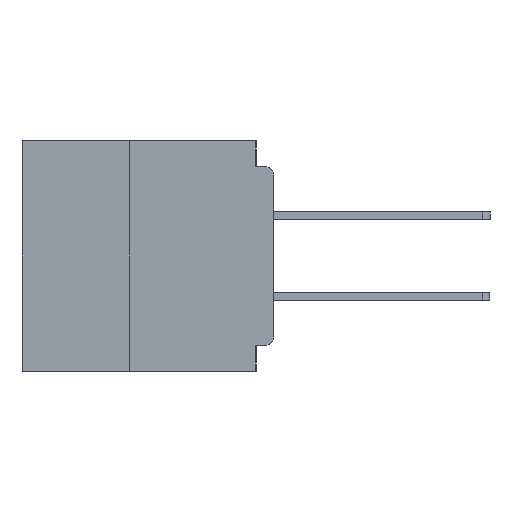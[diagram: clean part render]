
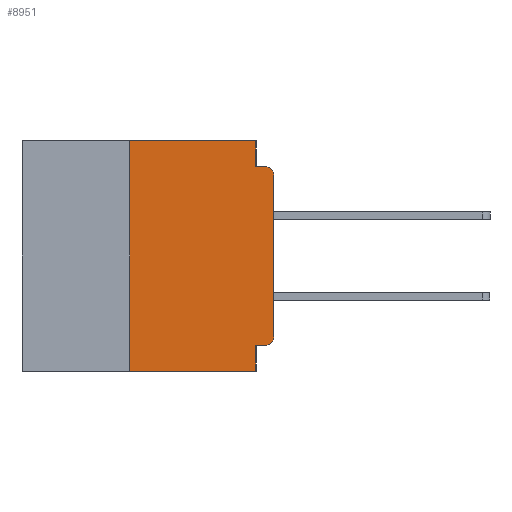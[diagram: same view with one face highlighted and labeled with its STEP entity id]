
A CAD part, left-side view. The second image highlights one B-rep face of the part: STEP entity #8951.
In plain terms, the highlighted planar face has unit normal (-1, 0, 0).
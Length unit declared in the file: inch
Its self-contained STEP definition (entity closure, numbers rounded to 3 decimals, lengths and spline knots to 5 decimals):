
#564 = DIRECTION ( 'NONE',  ( 0., -1., 0. ) ) ;
#827 = VERTEX_POINT ( 'NONE', #9445 ) ;
#1627 = VERTEX_POINT ( 'NONE', #43215 ) ;
#2192 = EDGE_CURVE ( 'NONE', #17711, #7327, #29854, .T. ) ;
#2783 = EDGE_CURVE ( 'NONE', #35785, #17711, #11024, .T. ) ;
#3082 = VECTOR ( 'NONE', #45607, 39.37008 ) ;
#7291 = ORIENTED_EDGE ( 'NONE', *, *, #34549, .F. ) ;
#7327 = VERTEX_POINT ( 'NONE', #21903 ) ;
#8363 = CARTESIAN_POINT ( 'NONE',  ( 0., 0.031, -0.355 ) ) ;
#8951 = ADVANCED_FACE ( 'NONE', ( #32500 ), #48819, .F. ) ;
#9445 = CARTESIAN_POINT ( 'NONE',  ( 0., 0.031, -0.045 ) ) ;
#10559 = VECTOR ( 'NONE', #37713, 39.37008 ) ;
#11024 = LINE ( 'NONE', #31619, #42430 ) ;
#11606 = EDGE_CURVE ( 'NONE', #52556, #18619, #43250, .T. ) ;
#11915 = CARTESIAN_POINT ( 'NONE',  ( 0., 0.437, 0. ) ) ;
#12272 = DIRECTION ( 'NONE',  ( 1., 0., 0. ) ) ;
#12718 = EDGE_CURVE ( 'NONE', #1627, #50601, #43747, .T. ) ;
#13626 = LINE ( 'NONE', #33648, #53060 ) ;
#14675 = VERTEX_POINT ( 'NONE', #44619 ) ;
#15361 = DIRECTION ( 'NONE',  ( 0., 0., 1. ) ) ;
#15692 = ORIENTED_EDGE ( 'NONE', *, *, #11606, .F. ) ;
#15844 = CARTESIAN_POINT ( 'NONE',  ( 0., 0.25, 0. ) ) ;
#17711 = VERTEX_POINT ( 'NONE', #30572 ) ;
#18619 = VERTEX_POINT ( 'NONE', #30398 ) ;
#20416 = CARTESIAN_POINT ( 'NONE',  ( 0., 0., -0.045 ) ) ;
#20626 = ORIENTED_EDGE ( 'NONE', *, *, #25111, .F. ) ;
#21029 = LINE ( 'NONE', #20416, #30584 ) ;
#21414 = LINE ( 'NONE', #23092, #42988 ) ;
#21698 = DIRECTION ( 'NONE',  ( -1., 0., 0. ) ) ;
#21903 = CARTESIAN_POINT ( 'NONE',  ( 0., 0.015, -0.045 ) ) ;
#22174 = VECTOR ( 'NONE', #15361, 39.37008 ) ;
#23092 = CARTESIAN_POINT ( 'NONE',  ( 0., 0., -0.355 ) ) ;
#24499 = EDGE_CURVE ( 'NONE', #50601, #25359, #13626, .T. ) ;
#25111 = EDGE_CURVE ( 'NONE', #25359, #827, #25230, .T. ) ;
#25230 = LINE ( 'NONE', #49822, #3082 ) ;
#25359 = VERTEX_POINT ( 'NONE', #51547 ) ;
#25375 = ORIENTED_EDGE ( 'NONE', *, *, #2783, .T. ) ;
#25551 = AXIS2_PLACEMENT_3D ( 'NONE', #11915, #12272, #40908 ) ;
#26894 = EDGE_CURVE ( 'NONE', #14675, #35785, #45286, .T. ) ;
#28307 = EDGE_CURVE ( 'NONE', #827, #7327, #21029, .T. ) ;
#29206 = VECTOR ( 'NONE', #30000, 39.37008 ) ;
#29854 = CIRCLE ( 'NONE', #42615, 0.015 ) ;
#29859 = EDGE_LOOP ( 'NONE', ( #25375, #40668, #43704, #20626, #52416, #32809, #48382, #15692, #7291, #38996 ) ) ;
#30000 = DIRECTION ( 'NONE',  ( 0., -1., 0. ) ) ;
#30398 = CARTESIAN_POINT ( 'NONE',  ( 0., 0.031, -0.4 ) ) ;
#30572 = CARTESIAN_POINT ( 'NONE',  ( 0., 0., -0.06 ) ) ;
#30584 = VECTOR ( 'NONE', #52757, 39.37008 ) ;
#31582 = DIRECTION ( 'NONE',  ( 0., 0., 1. ) ) ;
#31619 = CARTESIAN_POINT ( 'NONE',  ( 0., 0., 0. ) ) ;
#32500 = FACE_OUTER_BOUND ( 'NONE', #29859, .T. ) ;
#32809 = ORIENTED_EDGE ( 'NONE', *, *, #12718, .F. ) ;
#33648 = CARTESIAN_POINT ( 'NONE',  ( 0., 0.437, 0. ) ) ;
#33652 = CARTESIAN_POINT ( 'NONE',  ( 0., 0.031, -0.4 ) ) ;
#34549 = EDGE_CURVE ( 'NONE', #14675, #52556, #21414, .T. ) ;
#35204 = AXIS2_PLACEMENT_3D ( 'NONE', #45961, #21698, #50005 ) ;
#35780 = CARTESIAN_POINT ( 'NONE',  ( 0., 0.25, -0.4 ) ) ;
#35785 = VERTEX_POINT ( 'NONE', #44868 ) ;
#37713 = DIRECTION ( 'NONE',  ( 0., 0., -1. ) ) ;
#38996 = ORIENTED_EDGE ( 'NONE', *, *, #26894, .T. ) ;
#39945 = LINE ( 'NONE', #42020, #29206 ) ;
#40668 = ORIENTED_EDGE ( 'NONE', *, *, #2192, .T. ) ;
#40908 = DIRECTION ( 'NONE',  ( 0., 0., -1. ) ) ;
#42020 = CARTESIAN_POINT ( 'NONE',  ( 0., 0.437, -0.4 ) ) ;
#42430 = VECTOR ( 'NONE', #31582, 39.37008 ) ;
#42615 = AXIS2_PLACEMENT_3D ( 'NONE', #51393, #51164, #50764 ) ;
#42988 = VECTOR ( 'NONE', #51373, 39.37008 ) ;
#43215 = CARTESIAN_POINT ( 'NONE',  ( 0., 0.25, -0.4 ) ) ;
#43250 = LINE ( 'NONE', #33652, #10559 ) ;
#43704 = ORIENTED_EDGE ( 'NONE', *, *, #28307, .F. ) ;
#43747 = LINE ( 'NONE', #35780, #22174 ) ;
#44619 = CARTESIAN_POINT ( 'NONE',  ( 0., 0.015, -0.355 ) ) ;
#44868 = CARTESIAN_POINT ( 'NONE',  ( 0., 0., -0.34 ) ) ;
#45286 = CIRCLE ( 'NONE', #35204, 0.015 ) ;
#45607 = DIRECTION ( 'NONE',  ( 0., 0., -1. ) ) ;
#45961 = CARTESIAN_POINT ( 'NONE',  ( 0., 0.015, -0.34 ) ) ;
#47736 = EDGE_CURVE ( 'NONE', #1627, #18619, #39945, .T. ) ;
#48382 = ORIENTED_EDGE ( 'NONE', *, *, #47736, .T. ) ;
#48819 = PLANE ( 'NONE',  #25551 ) ;
#49822 = CARTESIAN_POINT ( 'NONE',  ( 0., 0.031, 0. ) ) ;
#50005 = DIRECTION ( 'NONE',  ( 0., 0., -1. ) ) ;
#50601 = VERTEX_POINT ( 'NONE', #15844 ) ;
#50764 = DIRECTION ( 'NONE',  ( 0., 0., -1. ) ) ;
#51164 = DIRECTION ( 'NONE',  ( -1., 0., 0. ) ) ;
#51373 = DIRECTION ( 'NONE',  ( 0., 1., 0. ) ) ;
#51393 = CARTESIAN_POINT ( 'NONE',  ( 0., 0.015, -0.06 ) ) ;
#51547 = CARTESIAN_POINT ( 'NONE',  ( 0., 0.031, 0. ) ) ;
#52416 = ORIENTED_EDGE ( 'NONE', *, *, #24499, .F. ) ;
#52556 = VERTEX_POINT ( 'NONE', #8363 ) ;
#52757 = DIRECTION ( 'NONE',  ( 0., -1., 0. ) ) ;
#53060 = VECTOR ( 'NONE', #564, 39.37008 ) ;
